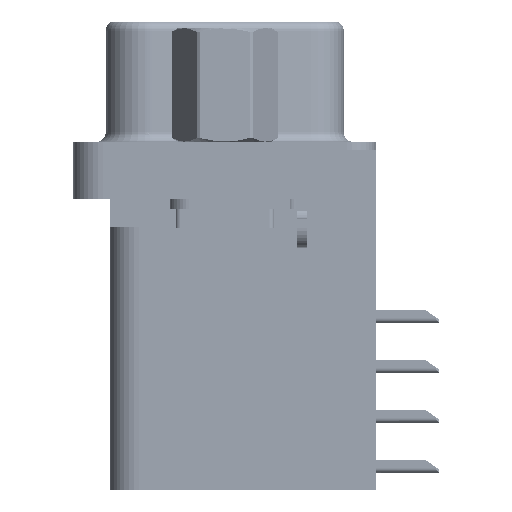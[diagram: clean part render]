
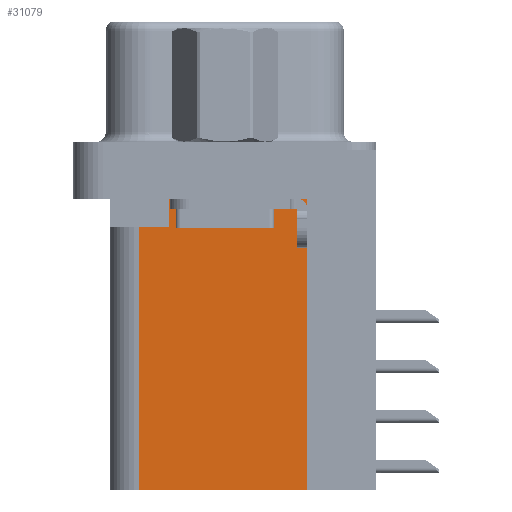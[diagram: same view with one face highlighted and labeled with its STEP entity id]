
A CAD part, left-side view. The second image highlights one B-rep face of the part: STEP entity #31079.
In plain terms, the highlighted planar face has unit normal (-1, 0, 0).
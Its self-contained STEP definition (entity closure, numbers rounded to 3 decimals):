
#1696 = ORIENTED_EDGE ( 'NONE', *, *, #17842, .F. ) ;
#4324 = VECTOR ( 'NONE', #11579, 1000. ) ;
#4549 = ORIENTED_EDGE ( 'NONE', *, *, #14014, .T. ) ;
#5182 = CARTESIAN_POINT ( 'NONE',  ( 3.75, 4.35, -17.3 ) ) ;
#5463 = LINE ( 'NONE', #7921, #4324 ) ;
#5549 = EDGE_CURVE ( 'NONE', #40359, #24123, #7154, .T. ) ;
#6016 = VECTOR ( 'NONE', #27233, 1000. ) ;
#7154 = LINE ( 'NONE', #44497, #6016 ) ;
#7921 = CARTESIAN_POINT ( 'NONE',  ( 3.75, 4.35, -17.3 ) ) ;
#9709 = ORIENTED_EDGE ( 'NONE', *, *, #5549, .T. ) ;
#11579 = DIRECTION ( 'NONE',  ( 0., 0., 1. ) ) ;
#12947 = ORIENTED_EDGE ( 'NONE', *, *, #25731, .F. ) ;
#13356 = DIRECTION ( 'NONE',  ( 0., 0., 1. ) ) ;
#14014 = EDGE_CURVE ( 'NONE', #44317, #24169, #18486, .T. ) ;
#14581 = CARTESIAN_POINT ( 'NONE',  ( 3.75, 2.85, -3.9 ) ) ;
#14663 = EDGE_CURVE ( 'NONE', #24123, #26862, #32166, .T. ) ;
#15728 = DIRECTION ( 'NONE',  ( 0., 1., 0. ) ) ;
#15845 = LINE ( 'NONE', #26304, #43606 ) ;
#16885 = CARTESIAN_POINT ( 'NONE',  ( 3.75, -4.2, -17.3 ) ) ;
#17842 = EDGE_CURVE ( 'NONE', #41079, #26862, #5463, .T. ) ;
#18486 = LINE ( 'NONE', #16885, #27293 ) ;
#19615 = VECTOR ( 'NONE', #44803, 1000. ) ;
#19916 = DIRECTION ( 'NONE',  ( 0., 1., 0. ) ) ;
#20016 = DIRECTION ( 'NONE',  ( 1., 0., 0. ) ) ;
#24123 = VERTEX_POINT ( 'NONE', #14581 ) ;
#24169 = VERTEX_POINT ( 'NONE', #32198 ) ;
#24289 = ORIENTED_EDGE ( 'NONE', *, *, #14663, .T. ) ;
#25731 = EDGE_CURVE ( 'NONE', #44317, #41079, #36795, .T. ) ;
#26304 = CARTESIAN_POINT ( 'NONE',  ( 3.75, -4.2, -2.5 ) ) ;
#26738 = CARTESIAN_POINT ( 'NONE',  ( 3.75, -4.2, -17.3 ) ) ;
#26862 = VERTEX_POINT ( 'NONE', #36311 ) ;
#27233 = DIRECTION ( 'NONE',  ( 0., 0., -1. ) ) ;
#27293 = VECTOR ( 'NONE', #13356, 1000. ) ;
#28458 = EDGE_CURVE ( 'NONE', #24169, #40359, #15845, .T. ) ;
#30084 = CARTESIAN_POINT ( 'NONE',  ( 3.75, 2.85, -2.5 ) ) ;
#31079 = ADVANCED_FACE ( 'NONE', ( #40629 ), #37329, .F. ) ;
#32166 = LINE ( 'NONE', #41315, #19615 ) ;
#32198 = CARTESIAN_POINT ( 'NONE',  ( 3.75, -4.2, -2.5 ) ) ;
#32883 = ORIENTED_EDGE ( 'NONE', *, *, #28458, .T. ) ;
#36311 = CARTESIAN_POINT ( 'NONE',  ( 3.75, 4.35, -3.9 ) ) ;
#36795 = LINE ( 'NONE', #26738, #44918 ) ;
#37283 = EDGE_LOOP ( 'NONE', ( #32883, #9709, #24289, #1696, #12947, #4549 ) ) ;
#37329 = PLANE ( 'NONE',  #39561 ) ;
#39462 = CARTESIAN_POINT ( 'NONE',  ( 3.75, -4.2, -17.3 ) ) ;
#39561 = AXIS2_PLACEMENT_3D ( 'NONE', #40788, #20016, #44283 ) ;
#40359 = VERTEX_POINT ( 'NONE', #30084 ) ;
#40629 = FACE_OUTER_BOUND ( 'NONE', #37283, .T. ) ;
#40788 = CARTESIAN_POINT ( 'NONE',  ( 3.75, -4.2, -17.3 ) ) ;
#41079 = VERTEX_POINT ( 'NONE', #5182 ) ;
#41315 = CARTESIAN_POINT ( 'NONE',  ( 3.75, 0., -3.9 ) ) ;
#43606 = VECTOR ( 'NONE', #15728, 1000. ) ;
#44283 = DIRECTION ( 'NONE',  ( 0., 1., 0. ) ) ;
#44317 = VERTEX_POINT ( 'NONE', #39462 ) ;
#44497 = CARTESIAN_POINT ( 'NONE',  ( 3.75, 2.85, -3.9 ) ) ;
#44803 = DIRECTION ( 'NONE',  ( 0., 1., 0. ) ) ;
#44918 = VECTOR ( 'NONE', #19916, 1000. ) ;
